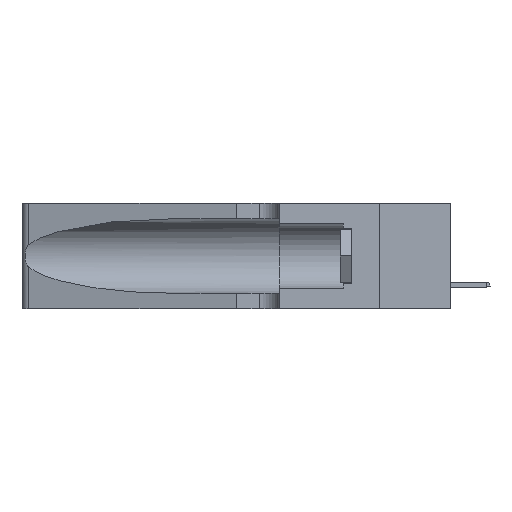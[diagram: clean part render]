
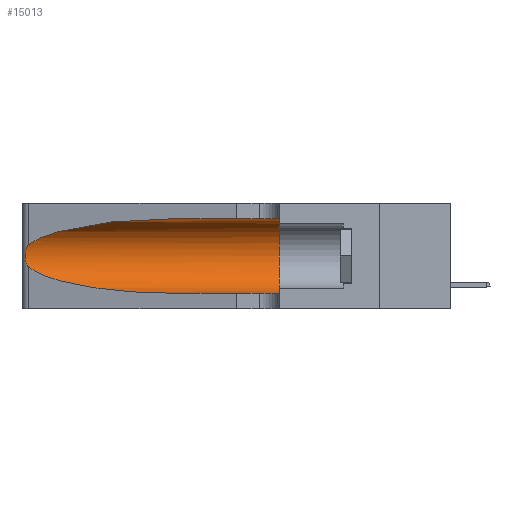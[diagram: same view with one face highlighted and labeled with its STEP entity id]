
A CAD part, left-side view. The second image highlights one B-rep face of the part: STEP entity #15013.
In plain terms, the highlighted cylindrical face has radius 3.308 mm (diameter 6.617 mm), a partial arc.
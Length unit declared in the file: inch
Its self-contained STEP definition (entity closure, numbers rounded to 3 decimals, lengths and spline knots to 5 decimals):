
#480 = DIRECTION ( 'NONE',  ( 0., 1., 0. ) ) ;
#1056 = CYLINDRICAL_SURFACE ( 'NONE', #8489, 0.13025 ) ;
#1461 = ORIENTED_EDGE ( 'NONE', *, *, #7516, .T. ) ;
#1697 = CARTESIAN_POINT ( 'NONE',  ( 0.25555, 1.22993, 0.14849 ) ) ;
#2095 = CARTESIAN_POINT ( 'NONE',  ( 0.26075, 1.23896, 0.178 ) ) ;
#2341 = DIRECTION ( 'NONE',  ( 0., -1., 0. ) ) ;
#2714 = CARTESIAN_POINT ( 'NONE',  ( 0.1305, 1.61858, 0.05475 ) ) ;
#3137 = CARTESIAN_POINT ( 'NONE',  ( 0.25487, 1.22718, 0.22369 ) ) ;
#3644 = VERTEX_POINT ( 'NONE', #15349 ) ;
#3807 = DIRECTION ( 'NONE',  ( 0., -1., 0. ) ) ;
#3951 = FACE_OUTER_BOUND ( 'NONE', #12897, .T. ) ;
#4275 = CARTESIAN_POINT ( 'NONE',  ( 0.18966, 0.96281, 0.31525 ) ) ;
#4778 = CARTESIAN_POINT ( 'NONE',  ( 0.25856, 1.23593, 0.16098 ) ) ;
#4964 = CARTESIAN_POINT ( 'NONE',  ( 0.25854, 1.2359, 0.20912 ) ) ;
#5157 = CIRCLE ( 'NONE', #15909, 0.13025 ) ;
#5779 = EDGE_CURVE ( 'NONE', #15925, #8447, #14186, .T. ) ;
#6243 = VERTEX_POINT ( 'NONE', #11550 ) ;
#6271 = VECTOR ( 'NONE', #3807, 39.37008 ) ;
#6473 = CARTESIAN_POINT ( 'NONE',  ( 0.25789, 1.23486, 0.15765 ) ) ;
#7516 = EDGE_CURVE ( 'NONE', #3644, #6243, #10239, .T. ) ;
#7629 = CARTESIAN_POINT ( 'NONE',  ( 0.25487, 1.22718, 0.22369 ) ) ;
#8447 = VERTEX_POINT ( 'NONE', #7629 ) ;
#8457 = EDGE_CURVE ( 'NONE', #8447, #3644, #8719, .T. ) ;
#8489 = AXIS2_PLACEMENT_3D ( 'NONE', #18855, #2341, #14244 ) ;
#8556 = DIRECTION ( 'NONE',  ( 0., -1., 0. ) ) ;
#8719 = B_SPLINE_CURVE_WITH_KNOTS ( 'NONE', 3,
 ( #3137, #13526, #15076, #9000, #4964, #14888, #12075, #2095, #9198, #4778, #6473, #17873, #1697, #13816 ),
 .UNSPECIFIED., .F., .F.,
 ( 4, 2, 2, 2, 2, 2, 4 ),
 ( 0., 0.00027, 0.00053, 0.00107, 0.0016, 0.00187, 0.00214 ),
 .UNSPECIFIED. ) ;
#8797 = CARTESIAN_POINT ( 'NONE',  ( 0.1305, 0.72297, 0.31525 ) ) ;
#9000 = CARTESIAN_POINT ( 'NONE',  ( 0.25787, 1.23484, 0.2124 ) ) ;
#9198 = CARTESIAN_POINT ( 'NONE',  ( 0.26017, 1.23833, 0.17102 ) ) ;
#9514 = DIRECTION ( 'NONE',  ( 0., 0., 1. ) ) ;
#9954 = CARTESIAN_POINT ( 'NONE',  ( 0.2373, 1.15595, 0.08982 ) ) ;
#10130 = CARTESIAN_POINT ( 'NONE',  ( 0.18966, 0.96281, 0.05475 ) ) ;
#10224 = CARTESIAN_POINT ( 'NONE',  ( 0.1305, 0.72297, 0.05475 ) ) ;
#10239 =( BOUNDED_CURVE ( )  B_SPLINE_CURVE ( 3, ( #11577, #9954, #10130, #10224 ),
 .UNSPECIFIED., .F., .F. ) 
 B_SPLINE_CURVE_WITH_KNOTS ( ( 4, 4 ),
 ( 3.44316, 4.71239 ),
 .UNSPECIFIED. ) 
 CURVE ( )  GEOMETRIC_REPRESENTATION_ITEM ( )  RATIONAL_B_SPLINE_CURVE ( ( 1., 0.87, 0.87, 1. ) ) 
 REPRESENTATION_ITEM ( '' )  );
#10574 = CARTESIAN_POINT ( 'NONE',  ( 0.1305, 0.35, 0.185 ) ) ;
#10907 = CARTESIAN_POINT ( 'NONE',  ( 0.1305, 0.35, 0.31525 ) ) ;
#11550 = CARTESIAN_POINT ( 'NONE',  ( 0.1305, 0.72297, 0.05475 ) ) ;
#11577 = CARTESIAN_POINT ( 'NONE',  ( 0.25487, 1.22718, 0.14631 ) ) ;
#12075 = CARTESIAN_POINT ( 'NONE',  ( 0.26075, 1.23896, 0.19203 ) ) ;
#12207 = ORIENTED_EDGE ( 'NONE', *, *, #5779, .T. ) ;
#12209 = ORIENTED_EDGE ( 'NONE', *, *, #15315, .F. ) ;
#12818 = EDGE_CURVE ( 'NONE', #15925, #13208, #16993, .T. ) ;
#12897 = EDGE_LOOP ( 'NONE', ( #12207, #12909, #1461, #18970, #12209, #15983 ) ) ;
#12909 = ORIENTED_EDGE ( 'NONE', *, *, #8457, .T. ) ;
#13091 = VECTOR ( 'NONE', #8556, 39.37008 ) ;
#13208 = VERTEX_POINT ( 'NONE', #10907 ) ;
#13225 = CARTESIAN_POINT ( 'NONE',  ( 0.25487, 1.22718, 0.22369 ) ) ;
#13526 = CARTESIAN_POINT ( 'NONE',  ( 0.25555, 1.22994, 0.2215 ) ) ;
#13816 = CARTESIAN_POINT ( 'NONE',  ( 0.25487, 1.22718, 0.14631 ) ) ;
#14186 =( BOUNDED_CURVE ( )  B_SPLINE_CURVE ( 3, ( #8797, #4275, #16023, #13225 ),
 .UNSPECIFIED., .F., .F. ) 
 B_SPLINE_CURVE_WITH_KNOTS ( ( 4, 4 ),
 ( 1.5708, 2.84003 ),
 .UNSPECIFIED. ) 
 CURVE ( )  GEOMETRIC_REPRESENTATION_ITEM ( )  RATIONAL_B_SPLINE_CURVE ( ( 1., 0.87, 0.87, 1. ) ) 
 REPRESENTATION_ITEM ( '' )  );
#14244 = DIRECTION ( 'NONE',  ( 0., 0., -1. ) ) ;
#14544 = LINE ( 'NONE', #2714, #13091 ) ;
#14663 = EDGE_CURVE ( 'NONE', #6243, #16884, #14544, .T. ) ;
#14766 = CARTESIAN_POINT ( 'NONE',  ( 0.1305, 0.35, 0.05475 ) ) ;
#14888 = CARTESIAN_POINT ( 'NONE',  ( 0.26018, 1.23835, 0.19895 ) ) ;
#15013 = ADVANCED_FACE ( 'NONE', ( #3951 ), #1056, .F. ) ;
#15076 = CARTESIAN_POINT ( 'NONE',  ( 0.25639, 1.23184, 0.21858 ) ) ;
#15315 = EDGE_CURVE ( 'NONE', #13208, #16884, #5157, .T. ) ;
#15349 = CARTESIAN_POINT ( 'NONE',  ( 0.25487, 1.22718, 0.14631 ) ) ;
#15909 = AXIS2_PLACEMENT_3D ( 'NONE', #10574, #480, #9514 ) ;
#15925 = VERTEX_POINT ( 'NONE', #17740 ) ;
#15983 = ORIENTED_EDGE ( 'NONE', *, *, #12818, .F. ) ;
#16023 = CARTESIAN_POINT ( 'NONE',  ( 0.2373, 1.15595, 0.28018 ) ) ;
#16884 = VERTEX_POINT ( 'NONE', #14766 ) ;
#16993 = LINE ( 'NONE', #18155, #6271 ) ;
#17740 = CARTESIAN_POINT ( 'NONE',  ( 0.1305, 0.72297, 0.31525 ) ) ;
#17873 = CARTESIAN_POINT ( 'NONE',  ( 0.25639, 1.23186, 0.15144 ) ) ;
#18155 = CARTESIAN_POINT ( 'NONE',  ( 0.1305, 1.61858, 0.31525 ) ) ;
#18855 = CARTESIAN_POINT ( 'NONE',  ( 0.1305, 1.61858, 0.185 ) ) ;
#18970 = ORIENTED_EDGE ( 'NONE', *, *, #14663, .T. ) ;
